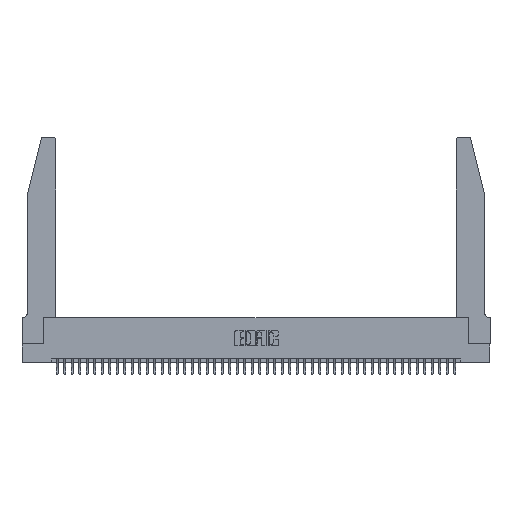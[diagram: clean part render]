
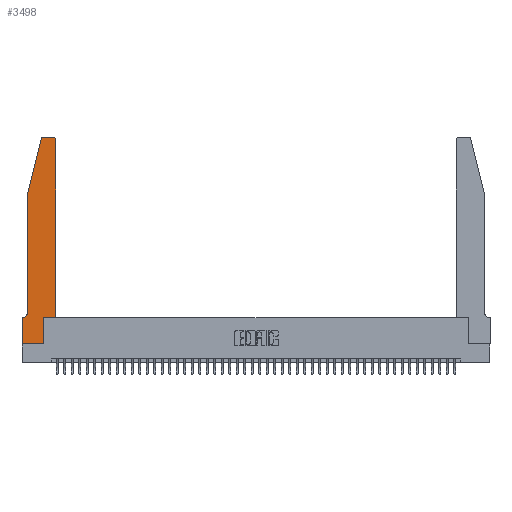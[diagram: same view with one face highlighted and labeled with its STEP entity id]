
A CAD part, top view. The second image highlights one B-rep face of the part: STEP entity #3498.
In plain terms, the highlighted planar face has unit normal (0, 0, 1).
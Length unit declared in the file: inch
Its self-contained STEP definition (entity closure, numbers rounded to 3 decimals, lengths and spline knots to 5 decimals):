
#247 = VECTOR ( 'NONE', #4794, 39.37008 ) ;
#1327 = CARTESIAN_POINT ( 'NONE',  ( 0.4205, 2.72, 0.37 ) ) ;
#1369 = ORIENTED_EDGE ( 'NONE', *, *, #23114, .T. ) ;
#1828 = CARTESIAN_POINT ( 'NONE',  ( 0.4505, 2.72, 0.37 ) ) ;
#1900 = VERTEX_POINT ( 'NONE', #34259 ) ;
#2285 = CARTESIAN_POINT ( 'NONE',  ( 0.2865, 0.35, 0.37 ) ) ;
#2904 = EDGE_CURVE ( 'NONE', #29928, #43266, #40974, .T. ) ;
#2963 = ORIENTED_EDGE ( 'NONE', *, *, #25374, .T. ) ;
#3141 = LINE ( 'NONE', #19262, #20300 ) ;
#3498 = ADVANCED_FACE ( 'NONE', ( #30001 ), #11911, .T. ) ;
#3684 = EDGE_CURVE ( 'NONE', #40838, #23597, #29951, .T. ) ;
#4007 = EDGE_CURVE ( 'NONE', #23597, #38142, #39826, .T. ) ;
#4256 = VERTEX_POINT ( 'NONE', #11131 ) ;
#4521 = CARTESIAN_POINT ( 'NONE',  ( 0.0755, 2., 0.37 ) ) ;
#4794 = DIRECTION ( 'NONE',  ( 0., -1., 0. ) ) ;
#5541 = LINE ( 'NONE', #22434, #32655 ) ;
#6477 = DIRECTION ( 'NONE',  ( 1., 0., 0. ) ) ;
#6939 = ORIENTED_EDGE ( 'NONE', *, *, #3684, .T. ) ;
#8734 = CARTESIAN_POINT ( 'NONE',  ( 0.4205, 2.75, 0.37 ) ) ;
#9302 = EDGE_CURVE ( 'NONE', #29520, #23649, #25214, .T. ) ;
#9887 = VERTEX_POINT ( 'NONE', #24827 ) ;
#11131 = CARTESIAN_POINT ( 'NONE',  ( 0., 0.35, 0.37 ) ) ;
#11471 = DIRECTION ( 'NONE',  ( 1., 0., 0. ) ) ;
#11665 = ORIENTED_EDGE ( 'NONE', *, *, #33588, .T. ) ;
#11911 = PLANE ( 'NONE',  #41130 ) ;
#11990 = DIRECTION ( 'NONE',  ( 0., -1., 0. ) ) ;
#12821 = VERTEX_POINT ( 'NONE', #42094 ) ;
#16101 = VECTOR ( 'NONE', #16132, 39.37008 ) ;
#16132 = DIRECTION ( 'NONE',  ( -0.239, -0.971, 0. ) ) ;
#16705 = VECTOR ( 'NONE', #39427, 39.37008 ) ;
#16707 = DIRECTION ( 'NONE',  ( -1., 0., 0. ) ) ;
#17430 = VECTOR ( 'NONE', #18441, 39.37008 ) ;
#18089 = LINE ( 'NONE', #24083, #35205 ) ;
#18441 = DIRECTION ( 'NONE',  ( 1., 0., 0. ) ) ;
#19051 = LINE ( 'NONE', #26010, #247 ) ;
#19071 = CARTESIAN_POINT ( 'NONE',  ( 0.0755, 2., 0.37 ) ) ;
#19219 = AXIS2_PLACEMENT_3D ( 'NONE', #1327, #36681, #6477 ) ;
#19262 = CARTESIAN_POINT ( 'NONE',  ( 0.4505, 0.35, 0.37 ) ) ;
#19353 = CIRCLE ( 'NONE', #26646, 0.07 ) ;
#19438 = LINE ( 'NONE', #25897, #16705 ) ;
#19787 = CARTESIAN_POINT ( 'NONE',  ( 0.0055, 0.42, 0.37 ) ) ;
#20241 = EDGE_CURVE ( 'NONE', #9887, #12821, #19353, .T. ) ;
#20299 = DIRECTION ( 'NONE',  ( 0., 0., 1. ) ) ;
#20300 = VECTOR ( 'NONE', #33037, 39.37008 ) ;
#20835 = CARTESIAN_POINT ( 'NONE',  ( 0.284, 2.75, 0.37 ) ) ;
#21299 = EDGE_CURVE ( 'NONE', #38142, #9887, #45200, .T. ) ;
#21308 = ORIENTED_EDGE ( 'NONE', *, *, #21908, .T. ) ;
#21807 = CARTESIAN_POINT ( 'NONE',  ( 0., 0.35, 0.37 ) ) ;
#21908 = EDGE_CURVE ( 'NONE', #12821, #4256, #18089, .T. ) ;
#22434 = CARTESIAN_POINT ( 'NONE',  ( 0., 0., 0.37 ) ) ;
#23008 = LINE ( 'NONE', #2285, #29065 ) ;
#23114 = EDGE_CURVE ( 'NONE', #4256, #28375, #19051, .T. ) ;
#23535 = EDGE_LOOP ( 'NONE', ( #2963, #6939, #33460, #31000, #33513, #21308, #1369, #30302, #29536, #45263, #11665, #25559 ) ) ;
#23597 = VERTEX_POINT ( 'NONE', #35793 ) ;
#23649 = VERTEX_POINT ( 'NONE', #42929 ) ;
#24083 = CARTESIAN_POINT ( 'NONE',  ( 0.0755, 0.35, 0.37 ) ) ;
#24827 = CARTESIAN_POINT ( 'NONE',  ( 0.0755, 0.42, 0.37 ) ) ;
#25214 = LINE ( 'NONE', #36028, #17430 ) ;
#25374 = EDGE_CURVE ( 'NONE', #43266, #40838, #19438, .T. ) ;
#25559 = ORIENTED_EDGE ( 'NONE', *, *, #2904, .T. ) ;
#25897 = CARTESIAN_POINT ( 'NONE',  ( 0.2605, 2.75, 0.37 ) ) ;
#26010 = CARTESIAN_POINT ( 'NONE',  ( 0., 0., 0.37 ) ) ;
#26128 = EDGE_CURVE ( 'NONE', #28375, #1900, #5541, .T. ) ;
#26646 = AXIS2_PLACEMENT_3D ( 'NONE', #19787, #44512, #16707 ) ;
#27264 = DIRECTION ( 'NONE',  ( 1., 0., 0. ) ) ;
#28375 = VERTEX_POINT ( 'NONE', #28860 ) ;
#28860 = CARTESIAN_POINT ( 'NONE',  ( 0., 0., 0.37 ) ) ;
#29065 = VECTOR ( 'NONE', #30453, 39.37008 ) ;
#29520 = VERTEX_POINT ( 'NONE', #44949 ) ;
#29536 = ORIENTED_EDGE ( 'NONE', *, *, #34703, .T. ) ;
#29928 = VERTEX_POINT ( 'NONE', #1828 ) ;
#29951 = CIRCLE ( 'NONE', #42919, 0.03 ) ;
#30001 = FACE_OUTER_BOUND ( 'NONE', #23535, .T. ) ;
#30302 = ORIENTED_EDGE ( 'NONE', *, *, #26128, .T. ) ;
#30453 = DIRECTION ( 'NONE',  ( 0., 1., 0. ) ) ;
#31000 = ORIENTED_EDGE ( 'NONE', *, *, #21299, .T. ) ;
#31664 = CARTESIAN_POINT ( 'NONE',  ( 0.0755, 2., 0.37 ) ) ;
#32655 = VECTOR ( 'NONE', #11471, 39.37008 ) ;
#33037 = DIRECTION ( 'NONE',  ( 0., 1., 0. ) ) ;
#33460 = ORIENTED_EDGE ( 'NONE', *, *, #4007, .T. ) ;
#33513 = ORIENTED_EDGE ( 'NONE', *, *, #20241, .T. ) ;
#33588 = EDGE_CURVE ( 'NONE', #23649, #29928, #3141, .T. ) ;
#34259 = CARTESIAN_POINT ( 'NONE',  ( 0.2865, 0., 0.37 ) ) ;
#34703 = EDGE_CURVE ( 'NONE', #1900, #29520, #23008, .T. ) ;
#35205 = VECTOR ( 'NONE', #44751, 39.37008 ) ;
#35793 = CARTESIAN_POINT ( 'NONE',  ( 0.25487, 2.72718, 0.37 ) ) ;
#36028 = CARTESIAN_POINT ( 'NONE',  ( 0.4505, 0.35, 0.37 ) ) ;
#36265 = DIRECTION ( 'NONE',  ( 0., 0., 1. ) ) ;
#36681 = DIRECTION ( 'NONE',  ( 0., 0., 1. ) ) ;
#38142 = VERTEX_POINT ( 'NONE', #4521 ) ;
#39427 = DIRECTION ( 'NONE',  ( -1., 0., 0. ) ) ;
#39826 = LINE ( 'NONE', #31664, #16101 ) ;
#39828 = DIRECTION ( 'NONE',  ( 1., 0., 0. ) ) ;
#40838 = VERTEX_POINT ( 'NONE', #20835 ) ;
#40974 = CIRCLE ( 'NONE', #19219, 0.03 ) ;
#41130 = AXIS2_PLACEMENT_3D ( 'NONE', #21807, #36265, #39828 ) ;
#41338 = VECTOR ( 'NONE', #11990, 39.37008 ) ;
#42094 = CARTESIAN_POINT ( 'NONE',  ( 0.0055, 0.35, 0.37 ) ) ;
#42919 = AXIS2_PLACEMENT_3D ( 'NONE', #44855, #20299, #27264 ) ;
#42929 = CARTESIAN_POINT ( 'NONE',  ( 0.4505, 0.35, 0.37 ) ) ;
#43266 = VERTEX_POINT ( 'NONE', #8734 ) ;
#44512 = DIRECTION ( 'NONE',  ( 0., 0., -1. ) ) ;
#44751 = DIRECTION ( 'NONE',  ( -1., 0., 0. ) ) ;
#44855 = CARTESIAN_POINT ( 'NONE',  ( 0.284, 2.72, 0.37 ) ) ;
#44949 = CARTESIAN_POINT ( 'NONE',  ( 0.2865, 0.35, 0.37 ) ) ;
#45200 = LINE ( 'NONE', #19071, #41338 ) ;
#45263 = ORIENTED_EDGE ( 'NONE', *, *, #9302, .T. ) ;
